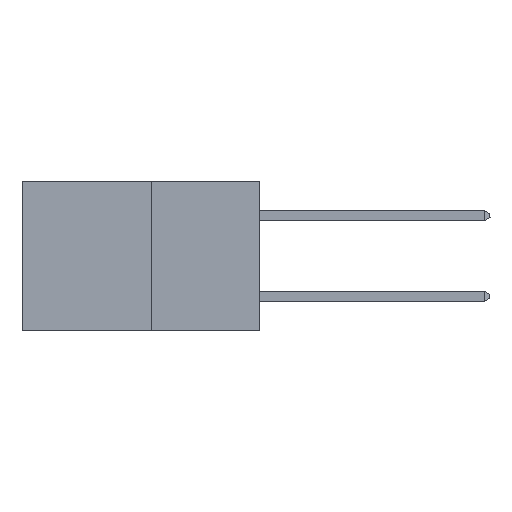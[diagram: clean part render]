
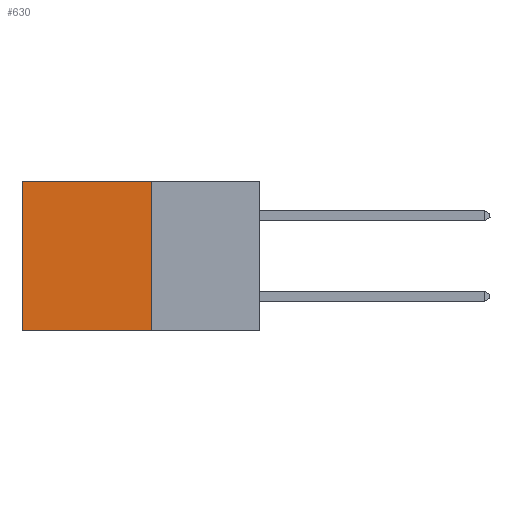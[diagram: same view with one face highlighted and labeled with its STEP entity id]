
A CAD part, left-side view. The second image highlights one B-rep face of the part: STEP entity #630.
In plain terms, the highlighted planar face has unit normal (-1, 0, 0).
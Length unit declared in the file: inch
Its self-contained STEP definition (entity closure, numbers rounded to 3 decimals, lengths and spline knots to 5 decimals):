
#128 = CARTESIAN_POINT ( 'NONE',  ( 0.277, 0.27, 0. ) ) ;
#630 = ADVANCED_FACE ( 'NONE', ( #4469 ), #18119, .F. ) ;
#795 = CARTESIAN_POINT ( 'NONE',  ( 0.277, 0.27, -0.37 ) ) ;
#841 = DIRECTION ( 'NONE',  ( 0., 1., 0. ) ) ;
#1982 = CARTESIAN_POINT ( 'NONE',  ( 0.277, 0.27, -0.37 ) ) ;
#2564 = ORIENTED_EDGE ( 'NONE', *, *, #17714, .F. ) ;
#3776 = ORIENTED_EDGE ( 'NONE', *, *, #17966, .T. ) ;
#4385 = VERTEX_POINT ( 'NONE', #7436 ) ;
#4469 = FACE_OUTER_BOUND ( 'NONE', #4502, .T. ) ;
#4476 = EDGE_CURVE ( 'NONE', #18568, #8148, #17289, .T. ) ;
#4502 = EDGE_LOOP ( 'NONE', ( #3776, #2564, #4851, #6539 ) ) ;
#4851 = ORIENTED_EDGE ( 'NONE', *, *, #9306, .F. ) ;
#6539 = ORIENTED_EDGE ( 'NONE', *, *, #4476, .T. ) ;
#6839 = VECTOR ( 'NONE', #14224, 39.37008 ) ;
#7436 = CARTESIAN_POINT ( 'NONE',  ( 0.277, 0.59, -0.37 ) ) ;
#8148 = VERTEX_POINT ( 'NONE', #9061 ) ;
#9061 = CARTESIAN_POINT ( 'NONE',  ( 0.277, 0.59, 0. ) ) ;
#9306 = EDGE_CURVE ( 'NONE', #18568, #15811, #19022, .T. ) ;
#9720 = CARTESIAN_POINT ( 'NONE',  ( 0.277, 0.27, 0. ) ) ;
#10946 = LINE ( 'NONE', #795, #11427 ) ;
#11427 = VECTOR ( 'NONE', #841, 39.37008 ) ;
#13736 = VECTOR ( 'NONE', #16441, 39.37008 ) ;
#14224 = DIRECTION ( 'NONE',  ( 0., 0., -1. ) ) ;
#15811 = VERTEX_POINT ( 'NONE', #19109 ) ;
#16441 = DIRECTION ( 'NONE',  ( 0., 0., -1. ) ) ;
#16814 = VECTOR ( 'NONE', #18783, 39.37008 ) ;
#17145 = CARTESIAN_POINT ( 'NONE',  ( 0.277, 0.59, -0.37 ) ) ;
#17289 = LINE ( 'NONE', #128, #16814 ) ;
#17512 = AXIS2_PLACEMENT_3D ( 'NONE', #18205, #18331, #18350 ) ;
#17714 = EDGE_CURVE ( 'NONE', #15811, #4385, #10946, .T. ) ;
#17851 = LINE ( 'NONE', #17145, #13736 ) ;
#17966 = EDGE_CURVE ( 'NONE', #8148, #4385, #17851, .T. ) ;
#18119 = PLANE ( 'NONE',  #17512 ) ;
#18205 = CARTESIAN_POINT ( 'NONE',  ( 0.277, 0.27, -0.37 ) ) ;
#18331 = DIRECTION ( 'NONE',  ( 1., 0., 0. ) ) ;
#18350 = DIRECTION ( 'NONE',  ( 0., 0., -1. ) ) ;
#18568 = VERTEX_POINT ( 'NONE', #9720 ) ;
#18783 = DIRECTION ( 'NONE',  ( 0., 1., 0. ) ) ;
#19022 = LINE ( 'NONE', #1982, #6839 ) ;
#19109 = CARTESIAN_POINT ( 'NONE',  ( 0.277, 0.27, -0.37 ) ) ;
